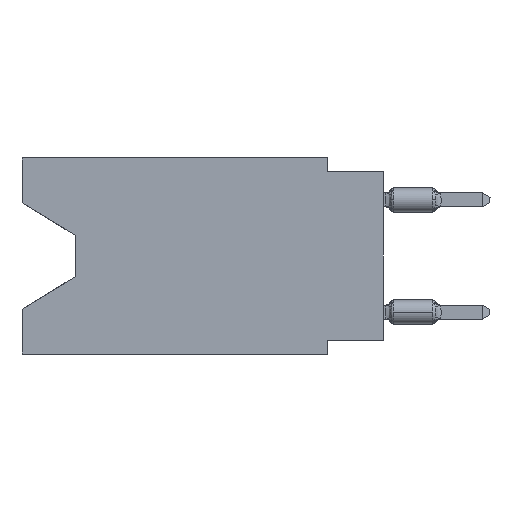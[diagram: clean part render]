
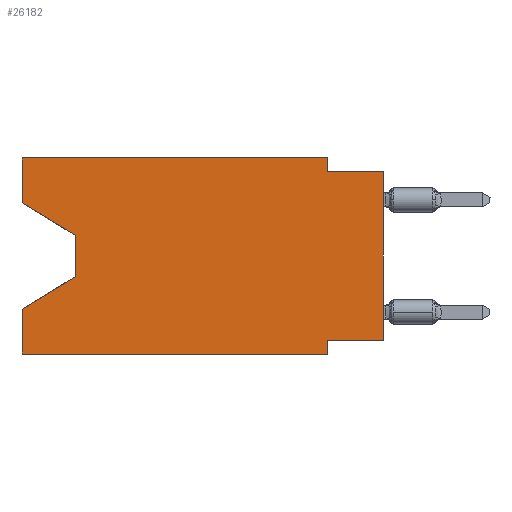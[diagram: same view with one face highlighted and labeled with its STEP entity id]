
A CAD part, left-side view. The second image highlights one B-rep face of the part: STEP entity #26182.
In plain terms, the highlighted planar face has unit normal (-1, 0, 0).
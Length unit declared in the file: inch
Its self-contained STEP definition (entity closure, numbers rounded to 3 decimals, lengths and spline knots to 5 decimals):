
#138 = ORIENTED_EDGE ( 'NONE', *, *, #4848, .F. ) ;
#336 = VECTOR ( 'NONE', #35379, 39.37008 ) ;
#854 = DIRECTION ( 'NONE',  ( 0., -0.855, -0.519 ) ) ;
#968 = VERTEX_POINT ( 'NONE', #15998 ) ;
#1858 = ORIENTED_EDGE ( 'NONE', *, *, #14326, .F. ) ;
#2368 = EDGE_CURVE ( 'NONE', #41488, #13030, #13445, .T. ) ;
#2590 = VECTOR ( 'NONE', #854, 39.37008 ) ;
#4848 = EDGE_CURVE ( 'NONE', #18571, #37127, #32277, .T. ) ;
#5573 = EDGE_LOOP ( 'NONE', ( #41806, #42552, #48954, #138, #39154, #33894, #47921, #15173, #45068, #6331, #1858, #51011 ) ) ;
#6319 = CARTESIAN_POINT ( 'NONE',  ( 0., 0.55, -0.138 ) ) ;
#6331 = ORIENTED_EDGE ( 'NONE', *, *, #9267, .F. ) ;
#6777 = EDGE_CURVE ( 'NONE', #41488, #49763, #9667, .T. ) ;
#6916 = LINE ( 'NONE', #11385, #19761 ) ;
#7035 = CARTESIAN_POINT ( 'NONE',  ( 0., 0.645, 0. ) ) ;
#8410 = LINE ( 'NONE', #17075, #25674 ) ;
#9267 = EDGE_CURVE ( 'NONE', #18582, #968, #21141, .T. ) ;
#9667 = LINE ( 'NONE', #37265, #34743 ) ;
#11385 = CARTESIAN_POINT ( 'NONE',  ( 0., 0.645, -0.35 ) ) ;
#11427 = LINE ( 'NONE', #19044, #19365 ) ;
#11541 = VERTEX_POINT ( 'NONE', #46038 ) ;
#12143 = EDGE_CURVE ( 'NONE', #51263, #17286, #51118, .T. ) ;
#13030 = VERTEX_POINT ( 'NONE', #28679 ) ;
#13445 = LINE ( 'NONE', #41035, #2590 ) ;
#13647 = CARTESIAN_POINT ( 'NONE',  ( 0., 0.645, 0. ) ) ;
#14326 = EDGE_CURVE ( 'NONE', #49763, #18582, #45439, .T. ) ;
#15173 = ORIENTED_EDGE ( 'NONE', *, *, #35135, .T. ) ;
#15998 = CARTESIAN_POINT ( 'NONE',  ( 0., 0.1, -0.025 ) ) ;
#17075 = CARTESIAN_POINT ( 'NONE',  ( 0., 0.55, -0.212 ) ) ;
#17286 = VERTEX_POINT ( 'NONE', #29342 ) ;
#18571 = VERTEX_POINT ( 'NONE', #42410 ) ;
#18582 = VERTEX_POINT ( 'NONE', #18738 ) ;
#18738 = CARTESIAN_POINT ( 'NONE',  ( 0., 0.1, 0. ) ) ;
#19044 = CARTESIAN_POINT ( 'NONE',  ( 0., 0., -0.025 ) ) ;
#19365 = VECTOR ( 'NONE', #43214, 39.37008 ) ;
#19498 = VECTOR ( 'NONE', #29689, 39.37008 ) ;
#19761 = VECTOR ( 'NONE', #22959, 39.37008 ) ;
#21141 = LINE ( 'NONE', #24041, #31134 ) ;
#22363 = DIRECTION ( 'NONE',  ( 0., 0., -1. ) ) ;
#22959 = DIRECTION ( 'NONE',  ( 0., -1., 0. ) ) ;
#23909 = DIRECTION ( 'NONE',  ( 1., 0., 0. ) ) ;
#24041 = CARTESIAN_POINT ( 'NONE',  ( 0., 0.1, 0. ) ) ;
#24452 = DIRECTION ( 'NONE',  ( 0., 0.855, -0.519 ) ) ;
#25156 = CARTESIAN_POINT ( 'NONE',  ( 0., 0., 0. ) ) ;
#25547 = VECTOR ( 'NONE', #38964, 39.37008 ) ;
#25674 = VECTOR ( 'NONE', #24452, 39.37008 ) ;
#26140 = EDGE_CURVE ( 'NONE', #13030, #45410, #42329, .T. ) ;
#26182 = ADVANCED_FACE ( 'NONE', ( #48057 ), #39667, .F. ) ;
#27094 = EDGE_CURVE ( 'NONE', #968, #47357, #11427, .T. ) ;
#27151 = CARTESIAN_POINT ( 'NONE',  ( 0., 0.1, -0.35 ) ) ;
#28340 = DIRECTION ( 'NONE',  ( 0., 0., 1. ) ) ;
#28679 = CARTESIAN_POINT ( 'NONE',  ( 0., 0.55, -0.138 ) ) ;
#29031 = DIRECTION ( 'NONE',  ( 0., 0., -1. ) ) ;
#29342 = CARTESIAN_POINT ( 'NONE',  ( 0., 0.1, -0.325 ) ) ;
#29655 = DIRECTION ( 'NONE',  ( 0., 0., 1. ) ) ;
#29689 = DIRECTION ( 'NONE',  ( 0., -1., 0. ) ) ;
#30456 = CARTESIAN_POINT ( 'NONE',  ( 0., 0., -0.025 ) ) ;
#30578 = LINE ( 'NONE', #27151, #25547 ) ;
#31098 = VECTOR ( 'NONE', #28340, 39.37008 ) ;
#31134 = VECTOR ( 'NONE', #29031, 39.37008 ) ;
#31704 = VECTOR ( 'NONE', #41175, 39.37008 ) ;
#31938 = AXIS2_PLACEMENT_3D ( 'NONE', #47285, #23909, #35733 ) ;
#32277 = LINE ( 'NONE', #48280, #31098 ) ;
#33894 = ORIENTED_EDGE ( 'NONE', *, *, #50958, .F. ) ;
#34743 = VECTOR ( 'NONE', #29655, 39.37008 ) ;
#35135 = EDGE_CURVE ( 'NONE', #51263, #47357, #45120, .T. ) ;
#35379 = DIRECTION ( 'NONE',  ( 0., 1., 0. ) ) ;
#35645 = CARTESIAN_POINT ( 'NONE',  ( 0., 0., -0.325 ) ) ;
#35733 = DIRECTION ( 'NONE',  ( 0., 0., -1. ) ) ;
#36037 = CARTESIAN_POINT ( 'NONE',  ( 0., 0.645, -0.26975 ) ) ;
#37104 = CARTESIAN_POINT ( 'NONE',  ( 0., 0., -0.325 ) ) ;
#37127 = VERTEX_POINT ( 'NONE', #36037 ) ;
#37265 = CARTESIAN_POINT ( 'NONE',  ( 0., 0.645, 0. ) ) ;
#38964 = DIRECTION ( 'NONE',  ( 0., 0., -1. ) ) ;
#39154 = ORIENTED_EDGE ( 'NONE', *, *, #49973, .T. ) ;
#39667 = PLANE ( 'NONE',  #31938 ) ;
#41035 = CARTESIAN_POINT ( 'NONE',  ( 0., 0.645, -0.08025 ) ) ;
#41175 = DIRECTION ( 'NONE',  ( 0., 0., 1. ) ) ;
#41488 = VERTEX_POINT ( 'NONE', #44413 ) ;
#41497 = EDGE_CURVE ( 'NONE', #45410, #37127, #8410, .T. ) ;
#41806 = ORIENTED_EDGE ( 'NONE', *, *, #2368, .T. ) ;
#42329 = LINE ( 'NONE', #6319, #42771 ) ;
#42410 = CARTESIAN_POINT ( 'NONE',  ( 0., 0.645, -0.35 ) ) ;
#42552 = ORIENTED_EDGE ( 'NONE', *, *, #26140, .T. ) ;
#42771 = VECTOR ( 'NONE', #22363, 39.37008 ) ;
#43214 = DIRECTION ( 'NONE',  ( 0., -1., 0. ) ) ;
#44413 = CARTESIAN_POINT ( 'NONE',  ( 0., 0.645, -0.08025 ) ) ;
#45068 = ORIENTED_EDGE ( 'NONE', *, *, #27094, .F. ) ;
#45120 = LINE ( 'NONE', #25156, #31704 ) ;
#45410 = VERTEX_POINT ( 'NONE', #45959 ) ;
#45439 = LINE ( 'NONE', #13647, #19498 ) ;
#45959 = CARTESIAN_POINT ( 'NONE',  ( 0., 0.55, -0.212 ) ) ;
#46038 = CARTESIAN_POINT ( 'NONE',  ( 0., 0.1, -0.35 ) ) ;
#47285 = CARTESIAN_POINT ( 'NONE',  ( 0., 0.645, 0. ) ) ;
#47357 = VERTEX_POINT ( 'NONE', #30456 ) ;
#47921 = ORIENTED_EDGE ( 'NONE', *, *, #12143, .F. ) ;
#48057 = FACE_OUTER_BOUND ( 'NONE', #5573, .T. ) ;
#48280 = CARTESIAN_POINT ( 'NONE',  ( 0., 0.645, 0. ) ) ;
#48954 = ORIENTED_EDGE ( 'NONE', *, *, #41497, .T. ) ;
#49763 = VERTEX_POINT ( 'NONE', #7035 ) ;
#49973 = EDGE_CURVE ( 'NONE', #18571, #11541, #6916, .T. ) ;
#50958 = EDGE_CURVE ( 'NONE', #17286, #11541, #30578, .T. ) ;
#51011 = ORIENTED_EDGE ( 'NONE', *, *, #6777, .F. ) ;
#51118 = LINE ( 'NONE', #35645, #336 ) ;
#51263 = VERTEX_POINT ( 'NONE', #37104 ) ;
